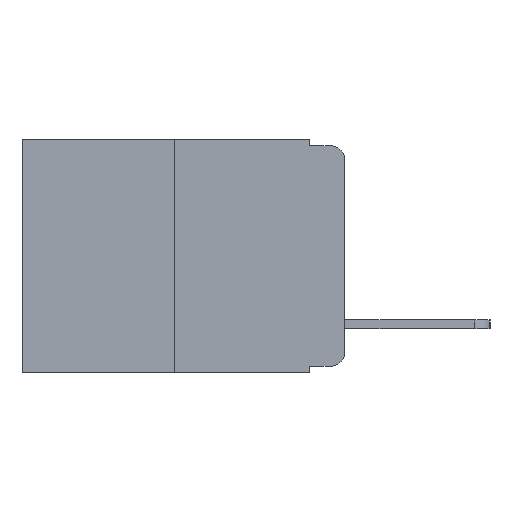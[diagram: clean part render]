
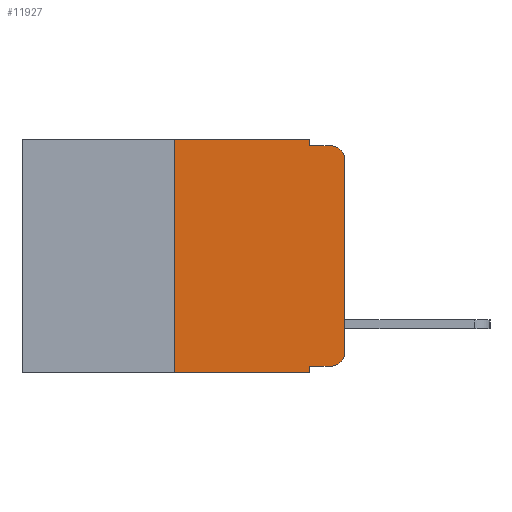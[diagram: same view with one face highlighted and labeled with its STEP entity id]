
A CAD part, left-side view. The second image highlights one B-rep face of the part: STEP entity #11927.
In plain terms, the highlighted planar face has unit normal (-1, 0, 0).
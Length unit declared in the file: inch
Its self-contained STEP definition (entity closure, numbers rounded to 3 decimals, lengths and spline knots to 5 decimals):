
#8 = EDGE_CURVE ( 'NONE', #8611, #12082, #13152, .T. ) ;
#42 = VERTEX_POINT ( 'NONE', #17293 ) ;
#92 = CARTESIAN_POINT ( 'NONE',  ( 0., 0.473, 0. ) ) ;
#730 = CIRCLE ( 'NONE', #6190, 0.02 ) ;
#1085 = FACE_OUTER_BOUND ( 'NONE', #17846, .T. ) ;
#1216 = AXIS2_PLACEMENT_3D ( 'NONE', #17735, #4189, #17707 ) ;
#1542 = LINE ( 'NONE', #23162, #20439 ) ;
#1689 = VERTEX_POINT ( 'NONE', #23110 ) ;
#1823 = DIRECTION ( 'NONE',  ( 0., 0., -1. ) ) ;
#1832 = LINE ( 'NONE', #8454, #15552 ) ;
#1979 = ORIENTED_EDGE ( 'NONE', *, *, #23508, .F. ) ;
#2237 = CARTESIAN_POINT ( 'NONE',  ( 0., 0.02, -0.01 ) ) ;
#2554 = LINE ( 'NONE', #16823, #16706 ) ;
#2566 = EDGE_CURVE ( 'NONE', #42, #10451, #1832, .T. ) ;
#2745 = CARTESIAN_POINT ( 'NONE',  ( 0., 0.02, -0.03 ) ) ;
#3474 = EDGE_CURVE ( 'NONE', #15749, #15920, #730, .T. ) ;
#4045 = LINE ( 'NONE', #8675, #21998 ) ;
#4189 = DIRECTION ( 'NONE',  ( -1., 0., 0. ) ) ;
#4285 = EDGE_CURVE ( 'NONE', #12082, #15749, #1542, .T. ) ;
#4307 = DIRECTION ( 'NONE',  ( 0., -1., 0. ) ) ;
#4734 = DIRECTION ( 'NONE',  ( 0., 0., -1. ) ) ;
#4754 = LINE ( 'NONE', #6878, #19664 ) ;
#5549 = CARTESIAN_POINT ( 'NONE',  ( 0., 0.051, -0.333 ) ) ;
#5588 = VERTEX_POINT ( 'NONE', #19495 ) ;
#5664 = ORIENTED_EDGE ( 'NONE', *, *, #3474, .T. ) ;
#5865 = CARTESIAN_POINT ( 'NONE',  ( 0., 0., -0.03 ) ) ;
#6190 = AXIS2_PLACEMENT_3D ( 'NONE', #2745, #15690, #4734 ) ;
#6323 = VERTEX_POINT ( 'NONE', #21710 ) ;
#6878 = CARTESIAN_POINT ( 'NONE',  ( 0., 0.051, -0.01 ) ) ;
#7436 = DIRECTION ( 'NONE',  ( 0., -1., 0. ) ) ;
#7995 = CARTESIAN_POINT ( 'NONE',  ( 0., 0.051, 0. ) ) ;
#8454 = CARTESIAN_POINT ( 'NONE',  ( 0., 0.473, -0.343 ) ) ;
#8610 = CARTESIAN_POINT ( 'NONE',  ( 0., 0.02, -0.333 ) ) ;
#8611 = VERTEX_POINT ( 'NONE', #8610 ) ;
#8675 = CARTESIAN_POINT ( 'NONE',  ( 0., 0.25, 0. ) ) ;
#10134 = LINE ( 'NONE', #21764, #14972 ) ;
#10451 = VERTEX_POINT ( 'NONE', #23704 ) ;
#10557 = DIRECTION ( 'NONE',  ( 0., -1., 0. ) ) ;
#11346 = CARTESIAN_POINT ( 'NONE',  ( 0., 0.473, 0. ) ) ;
#11731 = ORIENTED_EDGE ( 'NONE', *, *, #22367, .F. ) ;
#11927 = ADVANCED_FACE ( 'NONE', ( #1085 ), #16680, .F. ) ;
#12010 = VERTEX_POINT ( 'NONE', #7995 ) ;
#12082 = VERTEX_POINT ( 'NONE', #18681 ) ;
#12781 = DIRECTION ( 'NONE',  ( 0., 0., 1. ) ) ;
#13152 = CIRCLE ( 'NONE', #1216, 0.02 ) ;
#13187 = DIRECTION ( 'NONE',  ( 0., 0., -1. ) ) ;
#13207 = EDGE_CURVE ( 'NONE', #1689, #12010, #23498, .T. ) ;
#13764 = LINE ( 'NONE', #5549, #22382 ) ;
#14868 = ORIENTED_EDGE ( 'NONE', *, *, #13207, .F. ) ;
#14972 = VECTOR ( 'NONE', #1823, 39.37008 ) ;
#15075 = DIRECTION ( 'NONE',  ( 0., 0., -1. ) ) ;
#15409 = ORIENTED_EDGE ( 'NONE', *, *, #18917, .T. ) ;
#15552 = VECTOR ( 'NONE', #15736, 39.37008 ) ;
#15690 = DIRECTION ( 'NONE',  ( -1., 0., 0. ) ) ;
#15736 = DIRECTION ( 'NONE',  ( 0., -1., 0. ) ) ;
#15749 = VERTEX_POINT ( 'NONE', #5865 ) ;
#15920 = VERTEX_POINT ( 'NONE', #2237 ) ;
#16680 = PLANE ( 'NONE',  #17491 ) ;
#16706 = VECTOR ( 'NONE', #15075, 39.37008 ) ;
#16741 = ORIENTED_EDGE ( 'NONE', *, *, #4285, .T. ) ;
#16823 = CARTESIAN_POINT ( 'NONE',  ( 0., 0.051, 0. ) ) ;
#17058 = ORIENTED_EDGE ( 'NONE', *, *, #8, .T. ) ;
#17293 = CARTESIAN_POINT ( 'NONE',  ( 0., 0.25, -0.343 ) ) ;
#17491 = AXIS2_PLACEMENT_3D ( 'NONE', #11346, #23538, #13187 ) ;
#17707 = DIRECTION ( 'NONE',  ( 0., 0., -1. ) ) ;
#17735 = CARTESIAN_POINT ( 'NONE',  ( 0., 0.02, -0.313 ) ) ;
#17846 = EDGE_LOOP ( 'NONE', ( #16741, #5664, #18625, #22905, #14868, #11731, #20262, #1979, #15409, #17058 ) ) ;
#18625 = ORIENTED_EDGE ( 'NONE', *, *, #20783, .F. ) ;
#18681 = CARTESIAN_POINT ( 'NONE',  ( 0., 0., -0.313 ) ) ;
#18917 = EDGE_CURVE ( 'NONE', #6323, #8611, #13764, .T. ) ;
#19495 = CARTESIAN_POINT ( 'NONE',  ( 0., 0.051, -0.01 ) ) ;
#19664 = VECTOR ( 'NONE', #10557, 39.37008 ) ;
#20262 = ORIENTED_EDGE ( 'NONE', *, *, #2566, .T. ) ;
#20439 = VECTOR ( 'NONE', #12781, 39.37008 ) ;
#20783 = EDGE_CURVE ( 'NONE', #5588, #15920, #4754, .T. ) ;
#21060 = DIRECTION ( 'NONE',  ( 0., 0., 1. ) ) ;
#21234 = EDGE_CURVE ( 'NONE', #12010, #5588, #2554, .T. ) ;
#21710 = CARTESIAN_POINT ( 'NONE',  ( 0., 0.051, -0.333 ) ) ;
#21764 = CARTESIAN_POINT ( 'NONE',  ( 0., 0.051, 0. ) ) ;
#21998 = VECTOR ( 'NONE', #21060, 39.37008 ) ;
#22367 = EDGE_CURVE ( 'NONE', #42, #1689, #4045, .T. ) ;
#22382 = VECTOR ( 'NONE', #7436, 39.37008 ) ;
#22905 = ORIENTED_EDGE ( 'NONE', *, *, #21234, .F. ) ;
#22965 = VECTOR ( 'NONE', #4307, 39.37008 ) ;
#23110 = CARTESIAN_POINT ( 'NONE',  ( 0., 0.25, 0. ) ) ;
#23162 = CARTESIAN_POINT ( 'NONE',  ( 0., 0., 0. ) ) ;
#23498 = LINE ( 'NONE', #92, #22965 ) ;
#23508 = EDGE_CURVE ( 'NONE', #6323, #10451, #10134, .T. ) ;
#23538 = DIRECTION ( 'NONE',  ( 1., 0., 0. ) ) ;
#23704 = CARTESIAN_POINT ( 'NONE',  ( 0., 0.051, -0.343 ) ) ;
